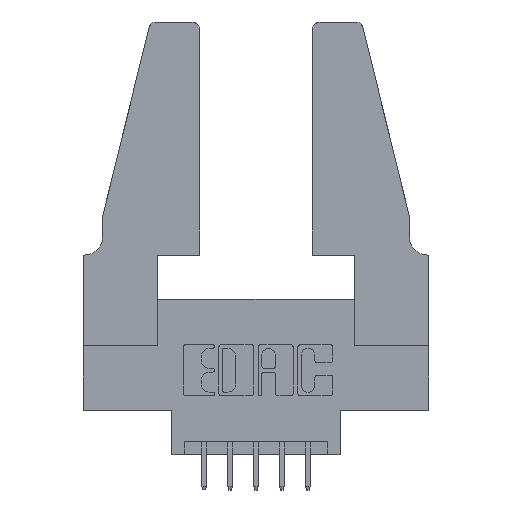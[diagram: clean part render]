
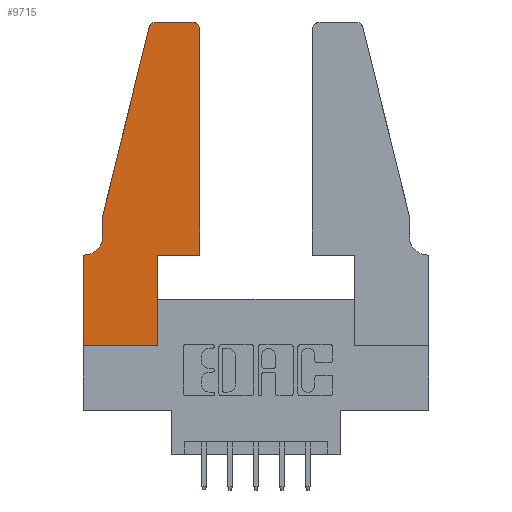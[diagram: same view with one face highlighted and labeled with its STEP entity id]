
A CAD part, top view. The second image highlights one B-rep face of the part: STEP entity #9715.
In plain terms, the highlighted planar face has unit normal (0, 0, 1).
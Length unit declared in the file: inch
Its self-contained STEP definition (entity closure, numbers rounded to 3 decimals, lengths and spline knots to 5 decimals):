
#42 = VERTEX_POINT ( 'NONE', #10881 ) ;
#114 = ORIENTED_EDGE ( 'NONE', *, *, #9992, .T. ) ;
#151 = CARTESIAN_POINT ( 'NONE',  ( 0.0755, 0.42, 0.37 ) ) ;
#459 = ORIENTED_EDGE ( 'NONE', *, *, #6679, .T. ) ;
#523 = VECTOR ( 'NONE', #5022, 39.37008 ) ;
#666 = DIRECTION ( 'NONE',  ( -0.239, -0.971, 0. ) ) ;
#696 = LINE ( 'NONE', #11105, #523 ) ;
#824 = CARTESIAN_POINT ( 'NONE',  ( 0., 0., 0.37 ) ) ;
#947 = DIRECTION ( 'NONE',  ( 0., 1., 0. ) ) ;
#998 = DIRECTION ( 'NONE',  ( -1., 0., 0. ) ) ;
#1081 = CARTESIAN_POINT ( 'NONE',  ( 0.2865, 0., 0.37 ) ) ;
#1503 = LINE ( 'NONE', #4972, #9128 ) ;
#1553 = CARTESIAN_POINT ( 'NONE',  ( 0., 0.35, 0.37 ) ) ;
#1601 = CARTESIAN_POINT ( 'NONE',  ( 0.0755, 0.35, 0.37 ) ) ;
#1789 = CARTESIAN_POINT ( 'NONE',  ( 0., 0.35, 0.37 ) ) ;
#1912 = EDGE_CURVE ( 'NONE', #5550, #2584, #696, .T. ) ;
#2063 = ORIENTED_EDGE ( 'NONE', *, *, #1912, .T. ) ;
#2075 = CARTESIAN_POINT ( 'NONE',  ( 0.4505, 1.22, 0.37 ) ) ;
#2318 = EDGE_CURVE ( 'NONE', #5717, #5550, #7643, .T. ) ;
#2329 = DIRECTION ( 'NONE',  ( 0., 0., 1. ) ) ;
#2368 = VECTOR ( 'NONE', #4768, 39.37008 ) ;
#2389 = LINE ( 'NONE', #10954, #3116 ) ;
#2545 = CARTESIAN_POINT ( 'NONE',  ( 0.0055, 0.35, 0.37 ) ) ;
#2584 = VERTEX_POINT ( 'NONE', #2075 ) ;
#2763 = DIRECTION ( 'NONE',  ( 0., 0., -1. ) ) ;
#2896 = CARTESIAN_POINT ( 'NONE',  ( 0.2605, 1.25, 0.37 ) ) ;
#3116 = VECTOR ( 'NONE', #666, 39.37008 ) ;
#3247 = DIRECTION ( 'NONE',  ( 1., 0., 0. ) ) ;
#3416 = ORIENTED_EDGE ( 'NONE', *, *, #8265, .T. ) ;
#3578 = CARTESIAN_POINT ( 'NONE',  ( 0.2865, 0.35, 0.37 ) ) ;
#4054 = LINE ( 'NONE', #1601, #7170 ) ;
#4093 = CARTESIAN_POINT ( 'NONE',  ( 0.284, 1.22, 0.37 ) ) ;
#4572 = FACE_OUTER_BOUND ( 'NONE', #9542, .T. ) ;
#4768 = DIRECTION ( 'NONE',  ( -1., 0., 0. ) ) ;
#4817 = LINE ( 'NONE', #824, #7952 ) ;
#4819 = VERTEX_POINT ( 'NONE', #1553 ) ;
#4858 = ORIENTED_EDGE ( 'NONE', *, *, #5764, .T. ) ;
#4972 = CARTESIAN_POINT ( 'NONE',  ( 0., 0., 0.37 ) ) ;
#5022 = DIRECTION ( 'NONE',  ( 0., 1., 0. ) ) ;
#5056 = AXIS2_PLACEMENT_3D ( 'NONE', #1789, #7071, #8853 ) ;
#5151 = DIRECTION ( 'NONE',  ( 1., 0., 0. ) ) ;
#5260 = CARTESIAN_POINT ( 'NONE',  ( 0.4205, 1.25, 0.37 ) ) ;
#5268 = LINE ( 'NONE', #3578, #6217 ) ;
#5412 = PLANE ( 'NONE',  #5056 ) ;
#5447 = LINE ( 'NONE', #9965, #10036 ) ;
#5550 = VERTEX_POINT ( 'NONE', #7359 ) ;
#5643 = ORIENTED_EDGE ( 'NONE', *, *, #10345, .T. ) ;
#5717 = VERTEX_POINT ( 'NONE', #9214 ) ;
#5764 = EDGE_CURVE ( 'NONE', #7454, #5785, #2389, .T. ) ;
#5785 = VERTEX_POINT ( 'NONE', #9341 ) ;
#5810 = EDGE_CURVE ( 'NONE', #42, #7454, #6210, .T. ) ;
#5812 = DIRECTION ( 'NONE',  ( -1., 0., 0. ) ) ;
#6050 = ORIENTED_EDGE ( 'NONE', *, *, #5810, .T. ) ;
#6065 = EDGE_CURVE ( 'NONE', #5785, #7444, #5447, .T. ) ;
#6210 = CIRCLE ( 'NONE', #9116, 0.03 ) ;
#6217 = VECTOR ( 'NONE', #947, 39.37008 ) ;
#6246 = CARTESIAN_POINT ( 'NONE',  ( 0.25487, 1.22718, 0.37 ) ) ;
#6300 = VERTEX_POINT ( 'NONE', #2545 ) ;
#6325 = EDGE_CURVE ( 'NONE', #7163, #5717, #5268, .T. ) ;
#6451 = ORIENTED_EDGE ( 'NONE', *, *, #2318, .T. ) ;
#6466 = DIRECTION ( 'NONE',  ( 0., -1., 0. ) ) ;
#6649 = ORIENTED_EDGE ( 'NONE', *, *, #6065, .T. ) ;
#6667 = CARTESIAN_POINT ( 'NONE',  ( 0., 0., 0.37 ) ) ;
#6679 = EDGE_CURVE ( 'NONE', #4819, #7792, #1503, .T. ) ;
#7071 = DIRECTION ( 'NONE',  ( 0., 0., 1. ) ) ;
#7136 = ORIENTED_EDGE ( 'NONE', *, *, #10564, .T. ) ;
#7163 = VERTEX_POINT ( 'NONE', #1081 ) ;
#7170 = VECTOR ( 'NONE', #5812, 39.37008 ) ;
#7211 = CIRCLE ( 'NONE', #8671, 0.07 ) ;
#7236 = LINE ( 'NONE', #2896, #2368 ) ;
#7282 = CIRCLE ( 'NONE', #10188, 0.03 ) ;
#7359 = CARTESIAN_POINT ( 'NONE',  ( 0.4505, 0.35, 0.37 ) ) ;
#7386 = DIRECTION ( 'NONE',  ( 0., -1., 0. ) ) ;
#7422 = DIRECTION ( 'NONE',  ( 1., 0., 0. ) ) ;
#7444 = VERTEX_POINT ( 'NONE', #151 ) ;
#7454 = VERTEX_POINT ( 'NONE', #6246 ) ;
#7464 = DIRECTION ( 'NONE',  ( 1., 0., 0. ) ) ;
#7475 = CARTESIAN_POINT ( 'NONE',  ( 0.4505, 0.35, 0.37 ) ) ;
#7643 = LINE ( 'NONE', #7475, #8018 ) ;
#7792 = VERTEX_POINT ( 'NONE', #6667 ) ;
#7952 = VECTOR ( 'NONE', #5151, 39.37008 ) ;
#8018 = VECTOR ( 'NONE', #7422, 39.37008 ) ;
#8265 = EDGE_CURVE ( 'NONE', #6300, #4819, #4054, .T. ) ;
#8671 = AXIS2_PLACEMENT_3D ( 'NONE', #8816, #2763, #998 ) ;
#8816 = CARTESIAN_POINT ( 'NONE',  ( 0.0055, 0.42, 0.37 ) ) ;
#8853 = DIRECTION ( 'NONE',  ( 1., 0., 0. ) ) ;
#9116 = AXIS2_PLACEMENT_3D ( 'NONE', #4093, #2329, #7464 ) ;
#9128 = VECTOR ( 'NONE', #7386, 39.37008 ) ;
#9214 = CARTESIAN_POINT ( 'NONE',  ( 0.2865, 0.35, 0.37 ) ) ;
#9341 = CARTESIAN_POINT ( 'NONE',  ( 0.0755, 0.5, 0.37 ) ) ;
#9395 = ORIENTED_EDGE ( 'NONE', *, *, #6325, .T. ) ;
#9542 = EDGE_LOOP ( 'NONE', ( #5643, #6050, #4858, #6649, #7136, #3416, #459, #11088, #9395, #6451, #2063, #114 ) ) ;
#9715 = ADVANCED_FACE ( 'NONE', ( #4572 ), #5412, .T. ) ;
#9965 = CARTESIAN_POINT ( 'NONE',  ( 0.0755, 0.5, 0.37 ) ) ;
#9992 = EDGE_CURVE ( 'NONE', #2584, #10632, #7282, .T. ) ;
#10036 = VECTOR ( 'NONE', #6466, 39.37008 ) ;
#10145 = CARTESIAN_POINT ( 'NONE',  ( 0.4205, 1.22, 0.37 ) ) ;
#10188 = AXIS2_PLACEMENT_3D ( 'NONE', #10145, #11081, #3247 ) ;
#10345 = EDGE_CURVE ( 'NONE', #10632, #42, #7236, .T. ) ;
#10477 = EDGE_CURVE ( 'NONE', #7792, #7163, #4817, .T. ) ;
#10564 = EDGE_CURVE ( 'NONE', #7444, #6300, #7211, .T. ) ;
#10632 = VERTEX_POINT ( 'NONE', #5260 ) ;
#10881 = CARTESIAN_POINT ( 'NONE',  ( 0.284, 1.25, 0.37 ) ) ;
#10954 = CARTESIAN_POINT ( 'NONE',  ( 0.0755, 0.5, 0.37 ) ) ;
#11081 = DIRECTION ( 'NONE',  ( 0., 0., 1. ) ) ;
#11088 = ORIENTED_EDGE ( 'NONE', *, *, #10477, .T. ) ;
#11105 = CARTESIAN_POINT ( 'NONE',  ( 0.4505, 0.35, 0.37 ) ) ;
